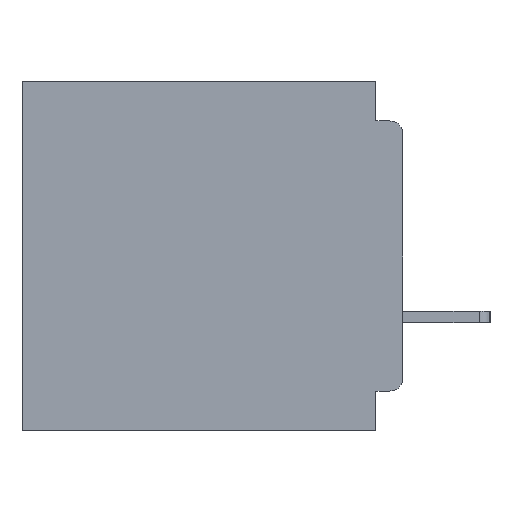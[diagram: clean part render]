
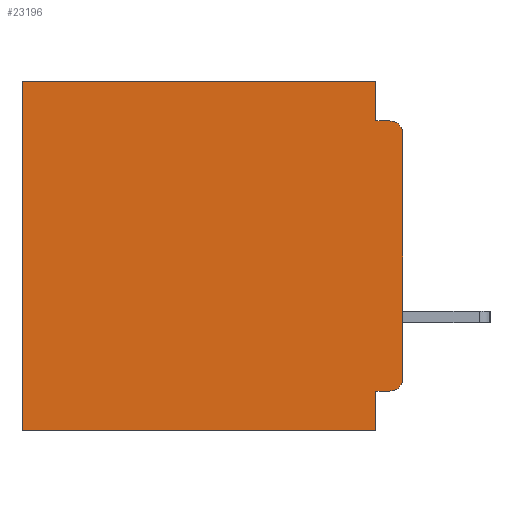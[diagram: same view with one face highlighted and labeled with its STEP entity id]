
A CAD part, left-side view. The second image highlights one B-rep face of the part: STEP entity #23196.
In plain terms, the highlighted planar face has unit normal (-1, 0, 0).
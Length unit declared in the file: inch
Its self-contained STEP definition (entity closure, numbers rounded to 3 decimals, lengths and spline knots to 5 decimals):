
#1151 = DIRECTION ( 'NONE',  ( -1., 0., 0. ) ) ;
#1883 = CARTESIAN_POINT ( 'NONE',  ( 0.3, 0.031, -0.355 ) ) ;
#2008 = LINE ( 'NONE', #6168, #19867 ) ;
#2822 = VERTEX_POINT ( 'NONE', #30978 ) ;
#2858 = ORIENTED_EDGE ( 'NONE', *, *, #19916, .F. ) ;
#3268 = AXIS2_PLACEMENT_3D ( 'NONE', #23945, #1151, #27742 ) ;
#4081 = LINE ( 'NONE', #41979, #11819 ) ;
#4703 = VECTOR ( 'NONE', #32102, 39.37008 ) ;
#4840 = PLANE ( 'NONE',  #35429 ) ;
#5229 = ORIENTED_EDGE ( 'NONE', *, *, #33605, .F. ) ;
#5336 = DIRECTION ( 'NONE',  ( -1., 0., 0. ) ) ;
#6168 = CARTESIAN_POINT ( 'NONE',  ( 0.3, 0.031, -0.4 ) ) ;
#6242 = VERTEX_POINT ( 'NONE', #18126 ) ;
#6318 = LINE ( 'NONE', #11604, #49036 ) ;
#7389 = CARTESIAN_POINT ( 'NONE',  ( 0.3, 0.437, -0.4 ) ) ;
#7538 = ORIENTED_EDGE ( 'NONE', *, *, #17003, .F. ) ;
#8183 = VECTOR ( 'NONE', #9811, 39.37008 ) ;
#8646 = DIRECTION ( 'NONE',  ( 0., 0., -1. ) ) ;
#9646 = CARTESIAN_POINT ( 'NONE',  ( 0.3, 0.031, -0.045 ) ) ;
#9787 = VERTEX_POINT ( 'NONE', #35350 ) ;
#9811 = DIRECTION ( 'NONE',  ( 0., 0., -1. ) ) ;
#10098 = CARTESIAN_POINT ( 'NONE',  ( 0.3, 0.437, 0. ) ) ;
#10855 = VERTEX_POINT ( 'NONE', #23301 ) ;
#11604 = CARTESIAN_POINT ( 'NONE',  ( 0.3, 0., 0. ) ) ;
#11819 = VECTOR ( 'NONE', #45757, 39.37008 ) ;
#13508 = VERTEX_POINT ( 'NONE', #43938 ) ;
#14941 = DIRECTION ( 'NONE',  ( 0., 0., -1. ) ) ;
#15779 = VERTEX_POINT ( 'NONE', #9646 ) ;
#16566 = FACE_OUTER_BOUND ( 'NONE', #49001, .T. ) ;
#16730 = VECTOR ( 'NONE', #25292, 39.37008 ) ;
#17003 = EDGE_CURVE ( 'NONE', #15779, #2822, #24901, .T. ) ;
#17799 = CIRCLE ( 'NONE', #3268, 0.015 ) ;
#18126 = CARTESIAN_POINT ( 'NONE',  ( 0.3, 0.015, -0.355 ) ) ;
#18466 = EDGE_CURVE ( 'NONE', #22585, #48244, #6318, .T. ) ;
#19460 = ORIENTED_EDGE ( 'NONE', *, *, #34483, .F. ) ;
#19867 = VECTOR ( 'NONE', #43999, 39.37008 ) ;
#19916 = EDGE_CURVE ( 'NONE', #22241, #38907, #2008, .T. ) ;
#19920 = AXIS2_PLACEMENT_3D ( 'NONE', #28086, #5336, #31907 ) ;
#20819 = CIRCLE ( 'NONE', #19920, 0.015 ) ;
#21002 = CARTESIAN_POINT ( 'NONE',  ( 0.3, 0., -0.045 ) ) ;
#22241 = VERTEX_POINT ( 'NONE', #1883 ) ;
#22585 = VERTEX_POINT ( 'NONE', #30709 ) ;
#22710 = EDGE_CURVE ( 'NONE', #9787, #2822, #17799, .T. ) ;
#22888 = VECTOR ( 'NONE', #32019, 39.37008 ) ;
#22916 = EDGE_CURVE ( 'NONE', #22585, #15779, #39721, .T. ) ;
#23194 = LINE ( 'NONE', #47985, #16730 ) ;
#23196 = ADVANCED_FACE ( 'NONE', ( #16566 ), #4840, .F. ) ;
#23301 = CARTESIAN_POINT ( 'NONE',  ( 0.3, 0., -0.34 ) ) ;
#23945 = CARTESIAN_POINT ( 'NONE',  ( 0.3, 0.015, -0.06 ) ) ;
#24819 = ORIENTED_EDGE ( 'NONE', *, *, #36894, .T. ) ;
#24901 = LINE ( 'NONE', #21002, #4703 ) ;
#25292 = DIRECTION ( 'NONE',  ( 0., 1., 0. ) ) ;
#26557 = ORIENTED_EDGE ( 'NONE', *, *, #22916, .F. ) ;
#27364 = EDGE_CURVE ( 'NONE', #6242, #10855, #20819, .T. ) ;
#27742 = DIRECTION ( 'NONE',  ( 0., 0., -1. ) ) ;
#28086 = CARTESIAN_POINT ( 'NONE',  ( 0.3, 0.015, -0.34 ) ) ;
#30709 = CARTESIAN_POINT ( 'NONE',  ( 0.3, 0.031, 0. ) ) ;
#30978 = CARTESIAN_POINT ( 'NONE',  ( 0.3, 0.015, -0.045 ) ) ;
#31397 = DIRECTION ( 'NONE',  ( 1., 0., 0. ) ) ;
#31907 = DIRECTION ( 'NONE',  ( 0., 0., -1. ) ) ;
#32019 = DIRECTION ( 'NONE',  ( 0., 1., 0. ) ) ;
#32102 = DIRECTION ( 'NONE',  ( 0., -1., 0. ) ) ;
#33605 = EDGE_CURVE ( 'NONE', #6242, #22241, #23194, .T. ) ;
#34483 = EDGE_CURVE ( 'NONE', #9787, #10855, #4081, .T. ) ;
#35350 = CARTESIAN_POINT ( 'NONE',  ( 0.3, 0., -0.06 ) ) ;
#35429 = AXIS2_PLACEMENT_3D ( 'NONE', #46446, #31397, #8646 ) ;
#36361 = CARTESIAN_POINT ( 'NONE',  ( 0.3, 0.031, -0.4 ) ) ;
#36894 = EDGE_CURVE ( 'NONE', #48244, #13508, #37058, .T. ) ;
#37058 = LINE ( 'NONE', #7389, #40091 ) ;
#38499 = ORIENTED_EDGE ( 'NONE', *, *, #48083, .F. ) ;
#38907 = VERTEX_POINT ( 'NONE', #36361 ) ;
#39721 = LINE ( 'NONE', #47605, #8183 ) ;
#40091 = VECTOR ( 'NONE', #14941, 39.37008 ) ;
#41975 = DIRECTION ( 'NONE',  ( 0., 1., 0. ) ) ;
#41979 = CARTESIAN_POINT ( 'NONE',  ( 0.3, 0., -0.4 ) ) ;
#41996 = ORIENTED_EDGE ( 'NONE', *, *, #22710, .T. ) ;
#43303 = CARTESIAN_POINT ( 'NONE',  ( 0.3, 0., -0.4 ) ) ;
#43804 = ORIENTED_EDGE ( 'NONE', *, *, #18466, .T. ) ;
#43938 = CARTESIAN_POINT ( 'NONE',  ( 0.3, 0.437, -0.4 ) ) ;
#43999 = DIRECTION ( 'NONE',  ( 0., 0., -1. ) ) ;
#44267 = LINE ( 'NONE', #43303, #22888 ) ;
#45757 = DIRECTION ( 'NONE',  ( 0., 0., -1. ) ) ;
#46446 = CARTESIAN_POINT ( 'NONE',  ( 0.3, 0., -0.4 ) ) ;
#46769 = ORIENTED_EDGE ( 'NONE', *, *, #27364, .T. ) ;
#47605 = CARTESIAN_POINT ( 'NONE',  ( 0.3, 0.031, 0. ) ) ;
#47985 = CARTESIAN_POINT ( 'NONE',  ( 0.3, 0., -0.355 ) ) ;
#48083 = EDGE_CURVE ( 'NONE', #38907, #13508, #44267, .T. ) ;
#48244 = VERTEX_POINT ( 'NONE', #10098 ) ;
#49001 = EDGE_LOOP ( 'NONE', ( #19460, #41996, #7538, #26557, #43804, #24819, #38499, #2858, #5229, #46769 ) ) ;
#49036 = VECTOR ( 'NONE', #41975, 39.37008 ) ;
